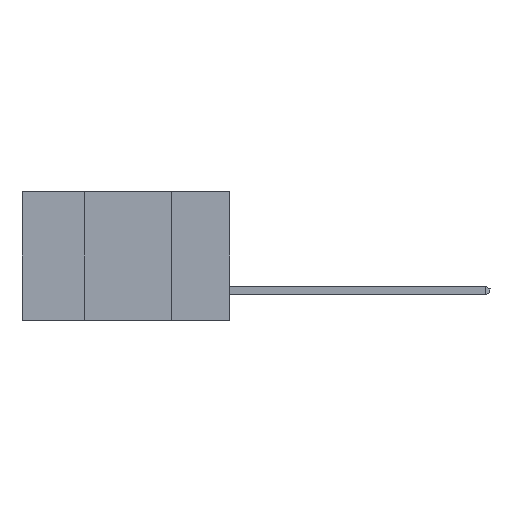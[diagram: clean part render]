
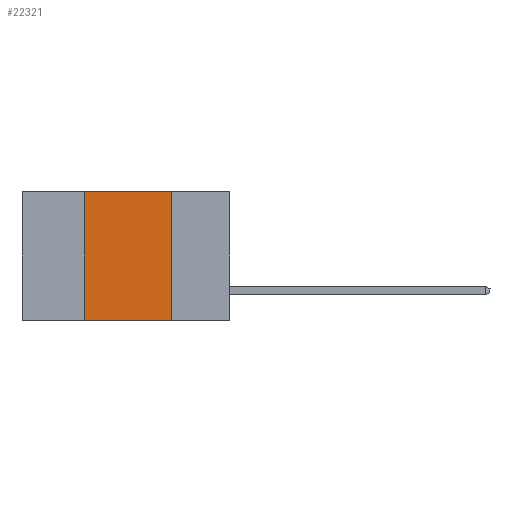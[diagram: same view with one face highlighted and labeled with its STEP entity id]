
A CAD part, left-side view. The second image highlights one B-rep face of the part: STEP entity #22321.
In plain terms, the highlighted planar face has unit normal (-1, 0, 0).
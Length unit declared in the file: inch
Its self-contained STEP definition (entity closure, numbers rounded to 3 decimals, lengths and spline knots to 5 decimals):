
#843 = DIRECTION ( 'NONE',  ( 0., 0., 1. ) ) ;
#1141 = CARTESIAN_POINT ( 'NONE',  ( 0., 0.17, -0.37 ) ) ;
#1262 = DIRECTION ( 'NONE',  ( 1., 0., 0. ) ) ;
#2887 = ORIENTED_EDGE ( 'NONE', *, *, #10653, .F. ) ;
#3452 = LINE ( 'NONE', #17211, #19701 ) ;
#3970 = VECTOR ( 'NONE', #23763, 39.37008 ) ;
#4345 = EDGE_CURVE ( 'NONE', #17244, #7101, #12941, .T. ) ;
#5183 = CARTESIAN_POINT ( 'NONE',  ( 0., 0.42, -0.37 ) ) ;
#6337 = CARTESIAN_POINT ( 'NONE',  ( 0., 0.42, 0. ) ) ;
#6953 = DIRECTION ( 'NONE',  ( 0., 0., -1. ) ) ;
#7101 = VERTEX_POINT ( 'NONE', #1141 ) ;
#8070 = EDGE_CURVE ( 'NONE', #14099, #17846, #9788, .T. ) ;
#9392 = DIRECTION ( 'NONE',  ( 0., 0., -1. ) ) ;
#9788 = LINE ( 'NONE', #19689, #3970 ) ;
#10653 = EDGE_CURVE ( 'NONE', #17244, #14099, #23127, .T. ) ;
#12499 = CARTESIAN_POINT ( 'NONE',  ( 0., 0.42, -0.37 ) ) ;
#12941 = LINE ( 'NONE', #18744, #17109 ) ;
#13174 = VECTOR ( 'NONE', #843, 39.37008 ) ;
#14099 = VERTEX_POINT ( 'NONE', #6337 ) ;
#16957 = CARTESIAN_POINT ( 'NONE',  ( 0., 0.17, 0. ) ) ;
#17109 = VECTOR ( 'NONE', #23071, 39.37008 ) ;
#17211 = CARTESIAN_POINT ( 'NONE',  ( 0., 0.17, -0.37 ) ) ;
#17244 = VERTEX_POINT ( 'NONE', #12499 ) ;
#17846 = VERTEX_POINT ( 'NONE', #16957 ) ;
#18249 = EDGE_LOOP ( 'NONE', ( #25109, #19039, #2887, #22819 ) ) ;
#18744 = CARTESIAN_POINT ( 'NONE',  ( 0., 0.6, -0.37 ) ) ;
#19039 = ORIENTED_EDGE ( 'NONE', *, *, #8070, .F. ) ;
#19352 = PLANE ( 'NONE',  #23351 ) ;
#19689 = CARTESIAN_POINT ( 'NONE',  ( 0., 0.6, 0. ) ) ;
#19701 = VECTOR ( 'NONE', #9392, 39.37008 ) ;
#21461 = CARTESIAN_POINT ( 'NONE',  ( 0., 0.6, 0. ) ) ;
#22321 = ADVANCED_FACE ( 'NONE', ( #25017 ), #19352, .F. ) ;
#22819 = ORIENTED_EDGE ( 'NONE', *, *, #4345, .T. ) ;
#23071 = DIRECTION ( 'NONE',  ( 0., -1., 0. ) ) ;
#23127 = LINE ( 'NONE', #5183, #13174 ) ;
#23351 = AXIS2_PLACEMENT_3D ( 'NONE', #21461, #1262, #6953 ) ;
#23763 = DIRECTION ( 'NONE',  ( 0., -1., 0. ) ) ;
#24827 = EDGE_CURVE ( 'NONE', #17846, #7101, #3452, .T. ) ;
#25017 = FACE_OUTER_BOUND ( 'NONE', #18249, .T. ) ;
#25109 = ORIENTED_EDGE ( 'NONE', *, *, #24827, .F. ) ;
